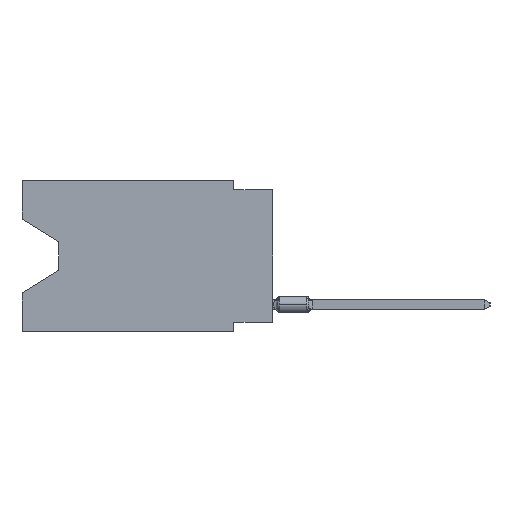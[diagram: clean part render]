
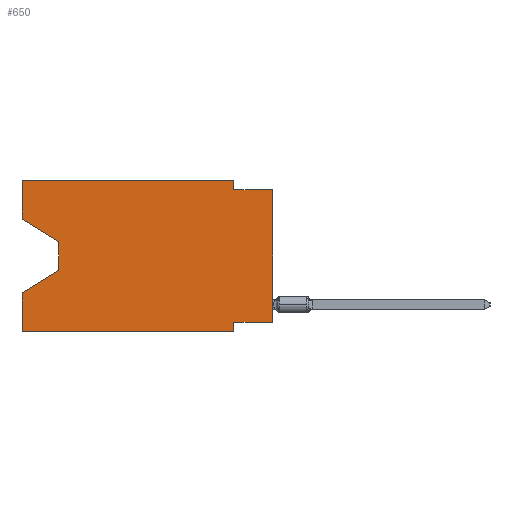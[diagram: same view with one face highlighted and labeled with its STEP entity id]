
A CAD part, left-side view. The second image highlights one B-rep face of the part: STEP entity #650.
In plain terms, the highlighted planar face has unit normal (-1, 0, 0).
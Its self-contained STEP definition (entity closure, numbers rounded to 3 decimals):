
#508 = VERTEX_POINT ( 'NONE', #8005 ) ;
#650 = ADVANCED_FACE ( 'NONE', ( #73853 ), #36004, .F. ) ;
#1813 = CARTESIAN_POINT ( 'NONE',  ( 0., 16.383, -2.546 ) ) ;
#2465 = LINE ( 'NONE', #13949, #19877 ) ;
#3581 = AXIS2_PLACEMENT_3D ( 'NONE', #73436, #48747, #35179 ) ;
#4139 = VERTEX_POINT ( 'NONE', #23200 ) ;
#6939 = CARTESIAN_POINT ( 'NONE',  ( 0., 13.97, -4.013 ) ) ;
#7689 = CARTESIAN_POINT ( 'NONE',  ( 0., 0., -0.635 ) ) ;
#7873 = CARTESIAN_POINT ( 'NONE',  ( 0., 16.383, 0. ) ) ;
#7992 = CARTESIAN_POINT ( 'NONE',  ( 0., 2.54, -9.271 ) ) ;
#8005 = CARTESIAN_POINT ( 'NONE',  ( 0., 2.54, -9.906 ) ) ;
#10584 = VECTOR ( 'NONE', #57498, 1000. ) ;
#10766 = VECTOR ( 'NONE', #58577, 1000. ) ;
#12508 = VECTOR ( 'NONE', #21764, 1000. ) ;
#12717 = CARTESIAN_POINT ( 'NONE',  ( 0., 16.383, -9.906 ) ) ;
#13949 = CARTESIAN_POINT ( 'NONE',  ( 0., 0., -0.635 ) ) ;
#14327 = EDGE_CURVE ( 'NONE', #37185, #68009, #58322, .T. ) ;
#15962 = EDGE_CURVE ( 'NONE', #64201, #38318, #66098, .T. ) ;
#16424 = CARTESIAN_POINT ( 'NONE',  ( 0., 16.383, -2.546 ) ) ;
#16944 = LINE ( 'NONE', #27726, #12508 ) ;
#17415 = VERTEX_POINT ( 'NONE', #45621 ) ;
#17885 = VERTEX_POINT ( 'NONE', #7689 ) ;
#18131 = EDGE_CURVE ( 'NONE', #64201, #508, #50127, .T. ) ;
#18766 = CARTESIAN_POINT ( 'NONE',  ( 0., 2.54, 0. ) ) ;
#19376 = DIRECTION ( 'NONE',  ( 0., 0., -1. ) ) ;
#19877 = VECTOR ( 'NONE', #78956, 1000. ) ;
#20522 = DIRECTION ( 'NONE',  ( 0., 0., -1. ) ) ;
#21044 = CARTESIAN_POINT ( 'NONE',  ( 0., 2.54, -9.906 ) ) ;
#21764 = DIRECTION ( 'NONE',  ( 0., 1., 0. ) ) ;
#23154 = ORIENTED_EDGE ( 'NONE', *, *, #15962, .F. ) ;
#23200 = CARTESIAN_POINT ( 'NONE',  ( 0., 13.97, -4.013 ) ) ;
#23769 = ORIENTED_EDGE ( 'NONE', *, *, #64586, .F. ) ;
#24741 = ORIENTED_EDGE ( 'NONE', *, *, #18131, .T. ) ;
#25295 = EDGE_CURVE ( 'NONE', #81631, #17885, #2465, .T. ) ;
#26489 = LINE ( 'NONE', #6939, #38488 ) ;
#27296 = ORIENTED_EDGE ( 'NONE', *, *, #25295, .F. ) ;
#27726 = CARTESIAN_POINT ( 'NONE',  ( 0., 0., -9.271 ) ) ;
#28264 = DIRECTION ( 'NONE',  ( 0., 0., 1. ) ) ;
#29978 = EDGE_CURVE ( 'NONE', #40524, #17885, #53045, .T. ) ;
#30195 = VERTEX_POINT ( 'NONE', #7992 ) ;
#30642 = VECTOR ( 'NONE', #28264, 1000. ) ;
#30645 = ORIENTED_EDGE ( 'NONE', *, *, #72412, .F. ) ;
#31202 = EDGE_CURVE ( 'NONE', #37185, #4139, #48298, .T. ) ;
#32784 = ORIENTED_EDGE ( 'NONE', *, *, #14327, .F. ) ;
#33340 = ORIENTED_EDGE ( 'NONE', *, *, #31202, .T. ) ;
#33467 = CARTESIAN_POINT ( 'NONE',  ( 0., 2.54, 0. ) ) ;
#34615 = CARTESIAN_POINT ( 'NONE',  ( 0., 16.383, 0. ) ) ;
#35146 = CARTESIAN_POINT ( 'NONE',  ( 0., 16.383, -9.906 ) ) ;
#35179 = DIRECTION ( 'NONE',  ( 0., 0., -1. ) ) ;
#35825 = ORIENTED_EDGE ( 'NONE', *, *, #59415, .F. ) ;
#36004 = PLANE ( 'NONE',  #3581 ) ;
#36694 = ORIENTED_EDGE ( 'NONE', *, *, #80190, .F. ) ;
#36979 = CARTESIAN_POINT ( 'NONE',  ( 0., 16.383, 0. ) ) ;
#37185 = VERTEX_POINT ( 'NONE', #1813 ) ;
#38205 = CARTESIAN_POINT ( 'NONE',  ( 0., 0., 0. ) ) ;
#38318 = VERTEX_POINT ( 'NONE', #67251 ) ;
#38488 = VECTOR ( 'NONE', #20522, 1000. ) ;
#38917 = LINE ( 'NONE', #21044, #53338 ) ;
#40137 = ORIENTED_EDGE ( 'NONE', *, *, #62637, .T. ) ;
#40524 = VERTEX_POINT ( 'NONE', #75354 ) ;
#40675 = VECTOR ( 'NONE', #77307, 1000. ) ;
#42344 = DIRECTION ( 'NONE',  ( 0., -0.855, -0.519 ) ) ;
#44410 = ORIENTED_EDGE ( 'NONE', *, *, #29978, .T. ) ;
#44688 = DIRECTION ( 'NONE',  ( 0., 0., -1. ) ) ;
#45159 = CARTESIAN_POINT ( 'NONE',  ( 0., 2.54, -0.635 ) ) ;
#45621 = CARTESIAN_POINT ( 'NONE',  ( 0., 13.97, -5.893 ) ) ;
#48298 = LINE ( 'NONE', #16424, #74689 ) ;
#48747 = DIRECTION ( 'NONE',  ( 1., 0., 0. ) ) ;
#50011 = LINE ( 'NONE', #68296, #73421 ) ;
#50127 = LINE ( 'NONE', #12717, #40675 ) ;
#52768 = EDGE_LOOP ( 'NONE', ( #33340, #83900, #40137, #23154, #24741, #23769, #30645, #44410, #27296, #35825, #36694, #32784 ) ) ;
#53045 = LINE ( 'NONE', #38205, #10766 ) ;
#53338 = VECTOR ( 'NONE', #19376, 1000. ) ;
#55677 = VERTEX_POINT ( 'NONE', #33467 ) ;
#57274 = VECTOR ( 'NONE', #44688, 1000. ) ;
#57498 = DIRECTION ( 'NONE',  ( 0., 0., 1. ) ) ;
#58322 = LINE ( 'NONE', #63887, #10584 ) ;
#58577 = DIRECTION ( 'NONE',  ( 0., 0., 1. ) ) ;
#59415 = EDGE_CURVE ( 'NONE', #55677, #81631, #76976, .T. ) ;
#60654 = VECTOR ( 'NONE', #79192, 1000. ) ;
#62637 = EDGE_CURVE ( 'NONE', #17415, #38318, #50011, .T. ) ;
#63887 = CARTESIAN_POINT ( 'NONE',  ( 0., 16.383, 0. ) ) ;
#64201 = VERTEX_POINT ( 'NONE', #35146 ) ;
#64586 = EDGE_CURVE ( 'NONE', #30195, #508, #38917, .T. ) ;
#64965 = EDGE_CURVE ( 'NONE', #4139, #17415, #26489, .T. ) ;
#66098 = LINE ( 'NONE', #7873, #30642 ) ;
#67251 = CARTESIAN_POINT ( 'NONE',  ( 0., 16.383, -7.36 ) ) ;
#68009 = VERTEX_POINT ( 'NONE', #34615 ) ;
#68296 = CARTESIAN_POINT ( 'NONE',  ( 0., 13.97, -5.893 ) ) ;
#69282 = LINE ( 'NONE', #36979, #60654 ) ;
#72412 = EDGE_CURVE ( 'NONE', #40524, #30195, #16944, .T. ) ;
#73421 = VECTOR ( 'NONE', #75940, 1000. ) ;
#73436 = CARTESIAN_POINT ( 'NONE',  ( 0., 16.383, 0. ) ) ;
#73853 = FACE_OUTER_BOUND ( 'NONE', #52768, .T. ) ;
#74689 = VECTOR ( 'NONE', #42344, 1000. ) ;
#75354 = CARTESIAN_POINT ( 'NONE',  ( 0., 0., -9.271 ) ) ;
#75940 = DIRECTION ( 'NONE',  ( 0., 0.855, -0.519 ) ) ;
#76976 = LINE ( 'NONE', #18766, #57274 ) ;
#77307 = DIRECTION ( 'NONE',  ( 0., -1., 0. ) ) ;
#78956 = DIRECTION ( 'NONE',  ( 0., -1., 0. ) ) ;
#79192 = DIRECTION ( 'NONE',  ( 0., -1., 0. ) ) ;
#80190 = EDGE_CURVE ( 'NONE', #68009, #55677, #69282, .T. ) ;
#81631 = VERTEX_POINT ( 'NONE', #45159 ) ;
#83900 = ORIENTED_EDGE ( 'NONE', *, *, #64965, .T. ) ;
